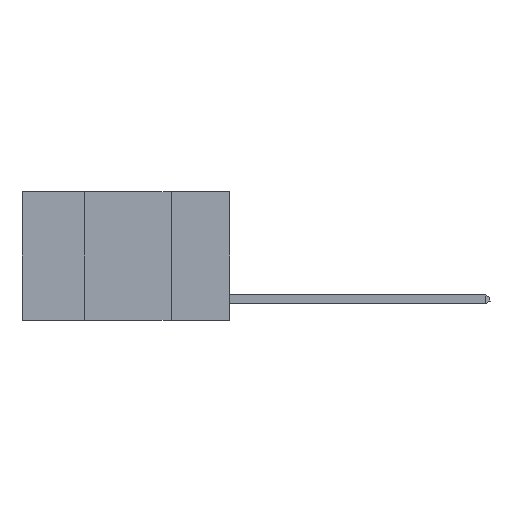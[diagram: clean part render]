
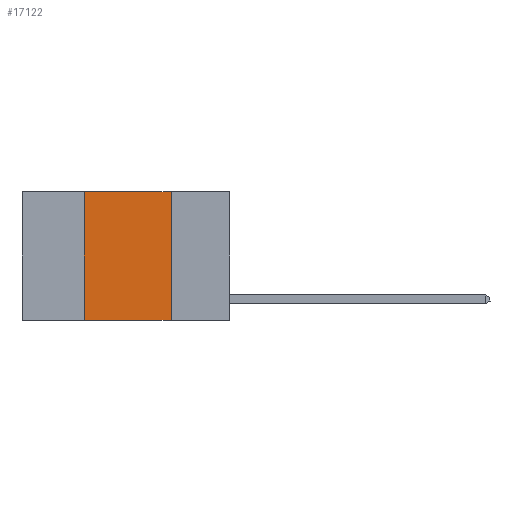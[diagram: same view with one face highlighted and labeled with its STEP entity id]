
A CAD part, left-side view. The second image highlights one B-rep face of the part: STEP entity #17122.
In plain terms, the highlighted planar face has unit normal (-1, 0, 0).
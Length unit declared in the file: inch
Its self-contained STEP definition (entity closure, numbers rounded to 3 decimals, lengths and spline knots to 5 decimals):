
#83 = VECTOR ( 'NONE', #3963, 39.37008 ) ;
#1464 = FACE_OUTER_BOUND ( 'NONE', #8659, .T. ) ;
#1655 = CARTESIAN_POINT ( 'NONE',  ( 0., 0.6, 0. ) ) ;
#1828 = VERTEX_POINT ( 'NONE', #7048 ) ;
#2507 = VERTEX_POINT ( 'NONE', #7581 ) ;
#3335 = ORIENTED_EDGE ( 'NONE', *, *, #3659, .T. ) ;
#3659 = EDGE_CURVE ( 'NONE', #2507, #10321, #7663, .T. ) ;
#3847 = PLANE ( 'NONE',  #10441 ) ;
#3963 = DIRECTION ( 'NONE',  ( 0., 0., 1. ) ) ;
#4131 = ORIENTED_EDGE ( 'NONE', *, *, #12077, .F. ) ;
#4569 = EDGE_CURVE ( 'NONE', #2507, #12510, #14212, .T. ) ;
#4654 = CARTESIAN_POINT ( 'NONE',  ( 0., 0.6, -0.37 ) ) ;
#4766 = DIRECTION ( 'NONE',  ( 0., -1., 0. ) ) ;
#5054 = VECTOR ( 'NONE', #16253, 39.37008 ) ;
#5165 = DIRECTION ( 'NONE',  ( 1., 0., 0. ) ) ;
#6925 = CARTESIAN_POINT ( 'NONE',  ( 0., 0.17, -0.37 ) ) ;
#7048 = CARTESIAN_POINT ( 'NONE',  ( 0., 0.17, 0. ) ) ;
#7254 = VECTOR ( 'NONE', #4766, 39.37008 ) ;
#7581 = CARTESIAN_POINT ( 'NONE',  ( 0., 0.42, -0.37 ) ) ;
#7663 = LINE ( 'NONE', #4654, #7254 ) ;
#8501 = LINE ( 'NONE', #1655, #5054 ) ;
#8659 = EDGE_LOOP ( 'NONE', ( #9728, #4131, #15733, #3335 ) ) ;
#8944 = EDGE_CURVE ( 'NONE', #1828, #10321, #16619, .T. ) ;
#9178 = VECTOR ( 'NONE', #9393, 39.37008 ) ;
#9393 = DIRECTION ( 'NONE',  ( 0., 0., -1. ) ) ;
#9728 = ORIENTED_EDGE ( 'NONE', *, *, #8944, .F. ) ;
#10321 = VERTEX_POINT ( 'NONE', #6925 ) ;
#10441 = AXIS2_PLACEMENT_3D ( 'NONE', #13027, #5165, #14340 ) ;
#11897 = CARTESIAN_POINT ( 'NONE',  ( 0., 0.42, 0. ) ) ;
#12013 = CARTESIAN_POINT ( 'NONE',  ( 0., 0.17, 0. ) ) ;
#12077 = EDGE_CURVE ( 'NONE', #12510, #1828, #8501, .T. ) ;
#12510 = VERTEX_POINT ( 'NONE', #11897 ) ;
#13027 = CARTESIAN_POINT ( 'NONE',  ( 0., 0.6, 0. ) ) ;
#14212 = LINE ( 'NONE', #14465, #83 ) ;
#14340 = DIRECTION ( 'NONE',  ( 0., 0., -1. ) ) ;
#14465 = CARTESIAN_POINT ( 'NONE',  ( 0., 0.42, 0. ) ) ;
#15733 = ORIENTED_EDGE ( 'NONE', *, *, #4569, .F. ) ;
#16253 = DIRECTION ( 'NONE',  ( 0., -1., 0. ) ) ;
#16619 = LINE ( 'NONE', #12013, #9178 ) ;
#17122 = ADVANCED_FACE ( 'NONE', ( #1464 ), #3847, .F. ) ;
